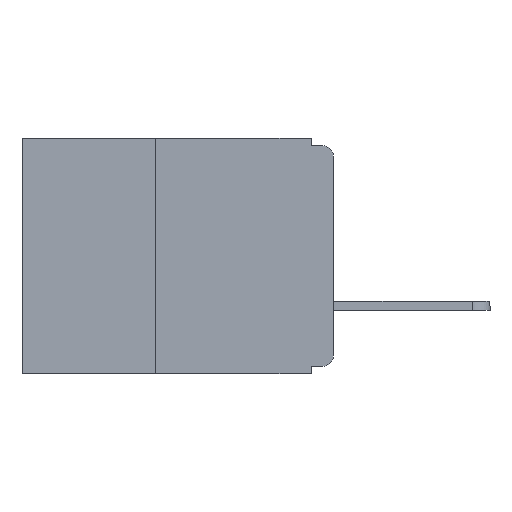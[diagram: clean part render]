
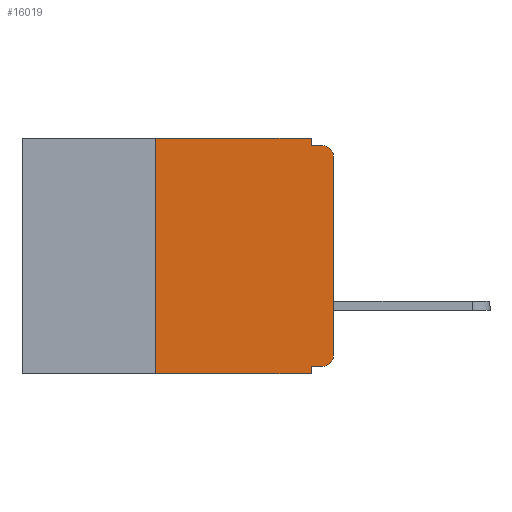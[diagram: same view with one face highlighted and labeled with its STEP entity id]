
A CAD part, left-side view. The second image highlights one B-rep face of the part: STEP entity #16019.
In plain terms, the highlighted planar face has unit normal (-1, 0, 0).
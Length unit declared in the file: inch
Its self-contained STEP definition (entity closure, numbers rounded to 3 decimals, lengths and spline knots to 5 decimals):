
#479 = VECTOR ( 'NONE', #3509, 39.37008 ) ;
#525 = CARTESIAN_POINT ( 'NONE',  ( 0., 0.031, 0. ) ) ;
#539 = DIRECTION ( 'NONE',  ( 1., 0., 0. ) ) ;
#607 = CARTESIAN_POINT ( 'NONE',  ( 0., 0., -0.025 ) ) ;
#635 = CARTESIAN_POINT ( 'NONE',  ( 0., 0.25, 0. ) ) ;
#905 = LINE ( 'NONE', #9587, #4239 ) ;
#1029 = CARTESIAN_POINT ( 'NONE',  ( 0., 0.015, -0.305 ) ) ;
#1036 = DIRECTION ( 'NONE',  ( 0., -1., 0. ) ) ;
#1451 = VERTEX_POINT ( 'NONE', #607 ) ;
#2193 = VERTEX_POINT ( 'NONE', #13236 ) ;
#2373 = ORIENTED_EDGE ( 'NONE', *, *, #19670, .F. ) ;
#2380 = AXIS2_PLACEMENT_3D ( 'NONE', #5109, #16646, #6761 ) ;
#2390 = LINE ( 'NONE', #9319, #11257 ) ;
#2673 = DIRECTION ( 'NONE',  ( 0., 0., -1. ) ) ;
#2697 = LINE ( 'NONE', #12420, #11030 ) ;
#2709 = EDGE_CURVE ( 'NONE', #15767, #19955, #11603, .T. ) ;
#3116 = AXIS2_PLACEMENT_3D ( 'NONE', #8811, #539, #12182 ) ;
#3509 = DIRECTION ( 'NONE',  ( 0., 0., 1. ) ) ;
#4239 = VECTOR ( 'NONE', #11281, 39.37008 ) ;
#4668 = ORIENTED_EDGE ( 'NONE', *, *, #2709, .F. ) ;
#5109 = CARTESIAN_POINT ( 'NONE',  ( 0., 0.015, -0.025 ) ) ;
#5265 = ORIENTED_EDGE ( 'NONE', *, *, #11025, .T. ) ;
#5398 = CARTESIAN_POINT ( 'NONE',  ( 0., 0.437, 0. ) ) ;
#5613 = VECTOR ( 'NONE', #16934, 39.37008 ) ;
#6761 = DIRECTION ( 'NONE',  ( 0., 0., -1. ) ) ;
#7166 = VECTOR ( 'NONE', #11919, 39.37008 ) ;
#7256 = ORIENTED_EDGE ( 'NONE', *, *, #10768, .F. ) ;
#7549 = VERTEX_POINT ( 'NONE', #635 ) ;
#8292 = CARTESIAN_POINT ( 'NONE',  ( 0., 0.015, -0.01 ) ) ;
#8811 = CARTESIAN_POINT ( 'NONE',  ( 0., 0.437, 0. ) ) ;
#9296 = LINE ( 'NONE', #16766, #479 ) ;
#9319 = CARTESIAN_POINT ( 'NONE',  ( 0., 0.031, 0. ) ) ;
#9587 = CARTESIAN_POINT ( 'NONE',  ( 0., 0., -0.32 ) ) ;
#9748 = LINE ( 'NONE', #16518, #17956 ) ;
#10430 = CIRCLE ( 'NONE', #2380, 0.015 ) ;
#10716 = DIRECTION ( 'NONE',  ( 0., 0., 1. ) ) ;
#10768 = EDGE_CURVE ( 'NONE', #11900, #17315, #2390, .T. ) ;
#10783 = VECTOR ( 'NONE', #1036, 39.37008 ) ;
#10884 = AXIS2_PLACEMENT_3D ( 'NONE', #1029, #12665, #2673 ) ;
#10979 = CARTESIAN_POINT ( 'NONE',  ( 0., 0.437, -0.33 ) ) ;
#11025 = EDGE_CURVE ( 'NONE', #1451, #11714, #10430, .T. ) ;
#11030 = VECTOR ( 'NONE', #10716, 39.37008 ) ;
#11257 = VECTOR ( 'NONE', #20804, 39.37008 ) ;
#11281 = DIRECTION ( 'NONE',  ( 0., 1., 0. ) ) ;
#11364 = EDGE_CURVE ( 'NONE', #21105, #2193, #17855, .T. ) ;
#11603 = LINE ( 'NONE', #11952, #7166 ) ;
#11714 = VERTEX_POINT ( 'NONE', #8292 ) ;
#11900 = VERTEX_POINT ( 'NONE', #525 ) ;
#11919 = DIRECTION ( 'NONE',  ( 0., 0., -1. ) ) ;
#11952 = CARTESIAN_POINT ( 'NONE',  ( 0., 0.031, -0.33 ) ) ;
#12016 = ORIENTED_EDGE ( 'NONE', *, *, #13243, .T. ) ;
#12182 = DIRECTION ( 'NONE',  ( 0., 0., -1. ) ) ;
#12420 = CARTESIAN_POINT ( 'NONE',  ( 0., 0.25, -0.33 ) ) ;
#12665 = DIRECTION ( 'NONE',  ( -1., 0., 0. ) ) ;
#12903 = EDGE_LOOP ( 'NONE', ( #12016, #5265, #18782, #7256, #21012, #2373, #15069, #4668, #17002, #14406 ) ) ;
#13236 = CARTESIAN_POINT ( 'NONE',  ( 0., 0., -0.305 ) ) ;
#13243 = EDGE_CURVE ( 'NONE', #2193, #1451, #9296, .T. ) ;
#14406 = ORIENTED_EDGE ( 'NONE', *, *, #11364, .T. ) ;
#14419 = EDGE_CURVE ( 'NONE', #17315, #11714, #9748, .T. ) ;
#14427 = CARTESIAN_POINT ( 'NONE',  ( 0., 0.031, -0.01 ) ) ;
#14782 = EDGE_CURVE ( 'NONE', #19938, #19955, #19458, .T. ) ;
#14893 = EDGE_CURVE ( 'NONE', #21105, #15767, #905, .T. ) ;
#14947 = DIRECTION ( 'NONE',  ( 0., -1., 0. ) ) ;
#15069 = ORIENTED_EDGE ( 'NONE', *, *, #14782, .T. ) ;
#15767 = VERTEX_POINT ( 'NONE', #21225 ) ;
#16019 = ADVANCED_FACE ( 'NONE', ( #18877 ), #20249, .F. ) ;
#16518 = CARTESIAN_POINT ( 'NONE',  ( 0., 0., -0.01 ) ) ;
#16646 = DIRECTION ( 'NONE',  ( -1., 0., 0. ) ) ;
#16766 = CARTESIAN_POINT ( 'NONE',  ( 0., 0., 0. ) ) ;
#16934 = DIRECTION ( 'NONE',  ( 0., -1., 0. ) ) ;
#17002 = ORIENTED_EDGE ( 'NONE', *, *, #14893, .F. ) ;
#17315 = VERTEX_POINT ( 'NONE', #14427 ) ;
#17855 = CIRCLE ( 'NONE', #10884, 0.015 ) ;
#17956 = VECTOR ( 'NONE', #14947, 39.37008 ) ;
#18230 = LINE ( 'NONE', #5398, #5613 ) ;
#18465 = CARTESIAN_POINT ( 'NONE',  ( 0., 0.031, -0.33 ) ) ;
#18490 = CARTESIAN_POINT ( 'NONE',  ( 0., 0.015, -0.32 ) ) ;
#18782 = ORIENTED_EDGE ( 'NONE', *, *, #14419, .F. ) ;
#18877 = FACE_OUTER_BOUND ( 'NONE', #12903, .T. ) ;
#19458 = LINE ( 'NONE', #10979, #10783 ) ;
#19670 = EDGE_CURVE ( 'NONE', #19938, #7549, #2697, .T. ) ;
#19938 = VERTEX_POINT ( 'NONE', #20871 ) ;
#19955 = VERTEX_POINT ( 'NONE', #18465 ) ;
#20249 = PLANE ( 'NONE',  #3116 ) ;
#20804 = DIRECTION ( 'NONE',  ( 0., 0., -1. ) ) ;
#20871 = CARTESIAN_POINT ( 'NONE',  ( 0., 0.25, -0.33 ) ) ;
#21012 = ORIENTED_EDGE ( 'NONE', *, *, #21107, .F. ) ;
#21105 = VERTEX_POINT ( 'NONE', #18490 ) ;
#21107 = EDGE_CURVE ( 'NONE', #7549, #11900, #18230, .T. ) ;
#21225 = CARTESIAN_POINT ( 'NONE',  ( 0., 0.031, -0.32 ) ) ;
